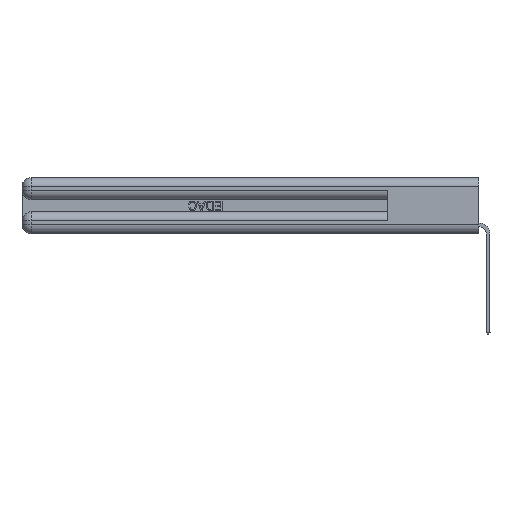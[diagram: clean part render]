
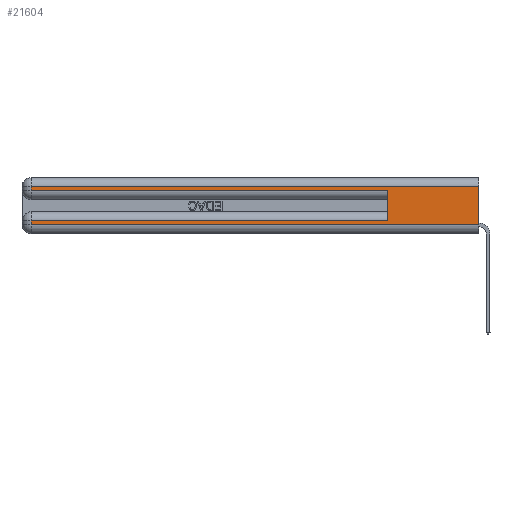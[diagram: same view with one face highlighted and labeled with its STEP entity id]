
A CAD part, left-side view. The second image highlights one B-rep face of the part: STEP entity #21604.
In plain terms, the highlighted planar face has unit normal (-1, 0, 0).
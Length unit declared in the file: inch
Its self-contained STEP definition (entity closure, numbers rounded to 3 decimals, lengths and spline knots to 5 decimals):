
#975 = EDGE_CURVE ( 'NONE', #1208, #16830, #12884, .T. ) ;
#1208 = VERTEX_POINT ( 'NONE', #11088 ) ;
#1313 = CARTESIAN_POINT ( 'NONE',  ( 0., 2.94, 0.085 ) ) ;
#2038 = ORIENTED_EDGE ( 'NONE', *, *, #21368, .T. ) ;
#2185 = CARTESIAN_POINT ( 'NONE',  ( 0., 0.6, 0.285 ) ) ;
#4274 = LINE ( 'NONE', #4636, #9947 ) ;
#4636 = CARTESIAN_POINT ( 'NONE',  ( 0., 0., 0.06 ) ) ;
#4970 = DIRECTION ( 'NONE',  ( 0., 1., 0. ) ) ;
#5142 = EDGE_CURVE ( 'NONE', #20959, #18891, #5448, .T. ) ;
#5448 = LINE ( 'NONE', #10087, #22364 ) ;
#5471 = VERTEX_POINT ( 'NONE', #1313 ) ;
#5945 = CARTESIAN_POINT ( 'NONE',  ( 0., 0., 0.085 ) ) ;
#6442 = VECTOR ( 'NONE', #14639, 39.37008 ) ;
#8946 = EDGE_CURVE ( 'NONE', #1208, #29067, #24020, .T. ) ;
#9740 = CARTESIAN_POINT ( 'NONE',  ( 0., 2.94, 0.06 ) ) ;
#9947 = VECTOR ( 'NONE', #20501, 39.37008 ) ;
#10087 = CARTESIAN_POINT ( 'NONE',  ( 0., 0.6, 0.145 ) ) ;
#10590 = CARTESIAN_POINT ( 'NONE',  ( 0., 2.94, 0.285 ) ) ;
#10852 = ORIENTED_EDGE ( 'NONE', *, *, #32199, .T. ) ;
#11088 = CARTESIAN_POINT ( 'NONE',  ( 0., 0., 0.31 ) ) ;
#12652 = DIRECTION ( 'NONE',  ( 0., 0., -1. ) ) ;
#12884 = LINE ( 'NONE', #26956, #21501 ) ;
#12996 = LINE ( 'NONE', #17830, #16508 ) ;
#13306 = ORIENTED_EDGE ( 'NONE', *, *, #31711, .T. ) ;
#14639 = DIRECTION ( 'NONE',  ( 0., 1., 0. ) ) ;
#14772 = VECTOR ( 'NONE', #28704, 39.37008 ) ;
#14983 = DIRECTION ( 'NONE',  ( 0., -1., 0. ) ) ;
#15091 = EDGE_CURVE ( 'NONE', #17174, #18891, #25490, .T. ) ;
#15520 = ORIENTED_EDGE ( 'NONE', *, *, #15091, .T. ) ;
#15539 = CARTESIAN_POINT ( 'NONE',  ( 0., 2.94, 0.37 ) ) ;
#16508 = VECTOR ( 'NONE', #12652, 39.37008 ) ;
#16830 = VERTEX_POINT ( 'NONE', #19724 ) ;
#17174 = VERTEX_POINT ( 'NONE', #10590 ) ;
#17315 = EDGE_LOOP ( 'NONE', ( #27193, #27156, #13306, #15520, #30542, #2038, #10852, #21945 ) ) ;
#17691 = DIRECTION ( 'NONE',  ( 0., 0., -1. ) ) ;
#17830 = CARTESIAN_POINT ( 'NONE',  ( 0., 2.94, 0.37 ) ) ;
#17861 = CARTESIAN_POINT ( 'NONE',  ( 0., 0., 0.37 ) ) ;
#18034 = PLANE ( 'NONE',  #28060 ) ;
#18891 = VERTEX_POINT ( 'NONE', #2185 ) ;
#19724 = CARTESIAN_POINT ( 'NONE',  ( 0., 0., 0.06 ) ) ;
#20501 = DIRECTION ( 'NONE',  ( 0., -1., 0. ) ) ;
#20520 = CARTESIAN_POINT ( 'NONE',  ( 0., 0., 0.285 ) ) ;
#20685 = VERTEX_POINT ( 'NONE', #9740 ) ;
#20959 = VERTEX_POINT ( 'NONE', #30883 ) ;
#21368 = EDGE_CURVE ( 'NONE', #20959, #5471, #22496, .T. ) ;
#21501 = VECTOR ( 'NONE', #23748, 39.37008 ) ;
#21604 = ADVANCED_FACE ( 'NONE', ( #33856 ), #18034, .F. ) ;
#21945 = ORIENTED_EDGE ( 'NONE', *, *, #23293, .T. ) ;
#22364 = VECTOR ( 'NONE', #31971, 39.37008 ) ;
#22496 = LINE ( 'NONE', #5945, #6442 ) ;
#23293 = EDGE_CURVE ( 'NONE', #20685, #16830, #4274, .T. ) ;
#23748 = DIRECTION ( 'NONE',  ( 0., 0., -1. ) ) ;
#24020 = LINE ( 'NONE', #32553, #32457 ) ;
#25490 = LINE ( 'NONE', #20520, #34072 ) ;
#26956 = CARTESIAN_POINT ( 'NONE',  ( 0., 0., 0.37 ) ) ;
#27156 = ORIENTED_EDGE ( 'NONE', *, *, #8946, .T. ) ;
#27193 = ORIENTED_EDGE ( 'NONE', *, *, #975, .F. ) ;
#28060 = AXIS2_PLACEMENT_3D ( 'NONE', #17861, #28349, #17691 ) ;
#28349 = DIRECTION ( 'NONE',  ( 1., 0., 0. ) ) ;
#28704 = DIRECTION ( 'NONE',  ( 0., 0., -1. ) ) ;
#29064 = LINE ( 'NONE', #15539, #14772 ) ;
#29067 = VERTEX_POINT ( 'NONE', #32980 ) ;
#30542 = ORIENTED_EDGE ( 'NONE', *, *, #5142, .F. ) ;
#30883 = CARTESIAN_POINT ( 'NONE',  ( 0., 0.6, 0.085 ) ) ;
#31711 = EDGE_CURVE ( 'NONE', #29067, #17174, #29064, .T. ) ;
#31971 = DIRECTION ( 'NONE',  ( 0., 0., 1. ) ) ;
#32199 = EDGE_CURVE ( 'NONE', #5471, #20685, #12996, .T. ) ;
#32457 = VECTOR ( 'NONE', #4970, 39.37008 ) ;
#32553 = CARTESIAN_POINT ( 'NONE',  ( 0., 0., 0.31 ) ) ;
#32980 = CARTESIAN_POINT ( 'NONE',  ( 0., 2.94, 0.31 ) ) ;
#33856 = FACE_OUTER_BOUND ( 'NONE', #17315, .T. ) ;
#34072 = VECTOR ( 'NONE', #14983, 39.37008 ) ;
